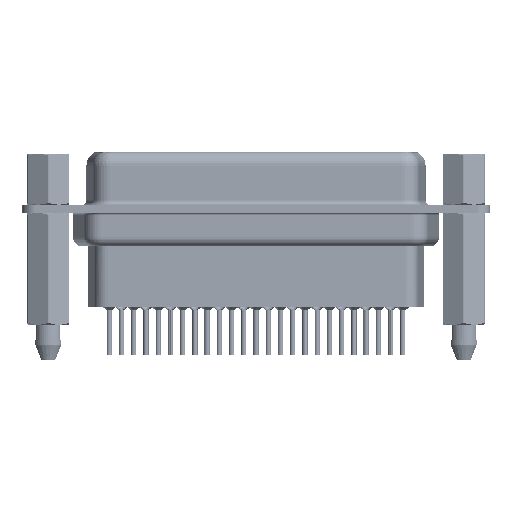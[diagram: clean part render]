
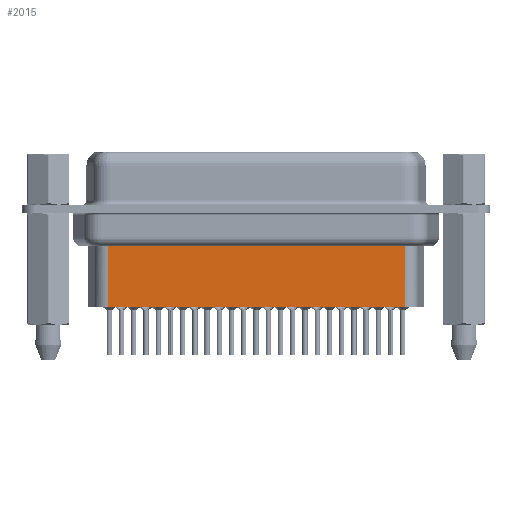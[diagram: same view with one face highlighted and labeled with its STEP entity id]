
A CAD part, front view. The second image highlights one B-rep face of the part: STEP entity #2015.
In plain terms, the highlighted planar face has unit normal (0, -1, 0).
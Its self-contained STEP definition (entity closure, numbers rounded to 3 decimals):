
#2015 = ADVANCED_FACE ( 'NONE', ( #13370 ), #20727, .T. ) ;
#3207 = VECTOR ( 'NONE', #32112, 1000. ) ;
#4141 = AXIS2_PLACEMENT_3D ( 'NONE', #31687, #5461, #31165 ) ;
#4623 = CARTESIAN_POINT ( 'NONE',  ( 6.706, -3.5, -4.097 ) ) ;
#5461 = DIRECTION ( 'NONE',  ( 0., -1., 0. ) ) ;
#7191 = VERTEX_POINT ( 'NONE', #22725 ) ;
#7336 = VECTOR ( 'NONE', #30791, 1000. ) ;
#8511 = DIRECTION ( 'NONE',  ( 0., 0., -1. ) ) ;
#10342 = EDGE_LOOP ( 'NONE', ( #32637, #25119, #26213, #14245 ) ) ;
#13370 = FACE_OUTER_BOUND ( 'NONE', #10342, .T. ) ;
#14245 = ORIENTED_EDGE ( 'NONE', *, *, #25553, .F. ) ;
#17457 = VERTEX_POINT ( 'NONE', #27431 ) ;
#19558 = VECTOR ( 'NONE', #24574, 1000. ) ;
#19754 = CARTESIAN_POINT ( 'NONE',  ( 6.706, -3.5, -11.15 ) ) ;
#19829 = EDGE_CURVE ( 'NONE', #23746, #27848, #27710, .T. ) ;
#20080 = EDGE_CURVE ( 'NONE', #27848, #17457, #31995, .T. ) ;
#20354 = CARTESIAN_POINT ( 'NONE',  ( 6.459, -3.5, -4.097 ) ) ;
#20727 = PLANE ( 'NONE',  #4141 ) ;
#21667 = LINE ( 'NONE', #29360, #3207 ) ;
#22411 = CARTESIAN_POINT ( 'NONE',  ( 40.344, -3.5, -4.097 ) ) ;
#22725 = CARTESIAN_POINT ( 'NONE',  ( 40.344, -3.5, -11.15 ) ) ;
#23746 = VERTEX_POINT ( 'NONE', #22411 ) ;
#24574 = DIRECTION ( 'NONE',  ( -1., 0., 0. ) ) ;
#25119 = ORIENTED_EDGE ( 'NONE', *, *, #19829, .T. ) ;
#25553 = EDGE_CURVE ( 'NONE', #7191, #17457, #32767, .T. ) ;
#26213 = ORIENTED_EDGE ( 'NONE', *, *, #20080, .T. ) ;
#26985 = EDGE_CURVE ( 'NONE', #23746, #7191, #21667, .T. ) ;
#27431 = CARTESIAN_POINT ( 'NONE',  ( 6.706, -3.5, -11.15 ) ) ;
#27710 = LINE ( 'NONE', #20354, #7336 ) ;
#27848 = VERTEX_POINT ( 'NONE', #4623 ) ;
#29360 = CARTESIAN_POINT ( 'NONE',  ( 40.344, -3.5, -3.1 ) ) ;
#29786 = VECTOR ( 'NONE', #8511, 1000. ) ;
#30791 = DIRECTION ( 'NONE',  ( -1., 0., 0. ) ) ;
#31165 = DIRECTION ( 'NONE',  ( 1., 0., 0. ) ) ;
#31687 = CARTESIAN_POINT ( 'NONE',  ( 6.706, -3.5, -3.1 ) ) ;
#31995 = LINE ( 'NONE', #32941, #29786 ) ;
#32112 = DIRECTION ( 'NONE',  ( 0., 0., -1. ) ) ;
#32637 = ORIENTED_EDGE ( 'NONE', *, *, #26985, .F. ) ;
#32767 = LINE ( 'NONE', #19754, #19558 ) ;
#32941 = CARTESIAN_POINT ( 'NONE',  ( 6.706, -3.5, -3.1 ) ) ;
